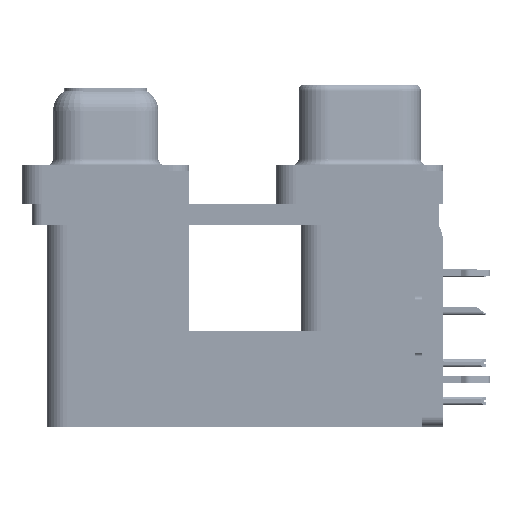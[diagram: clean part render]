
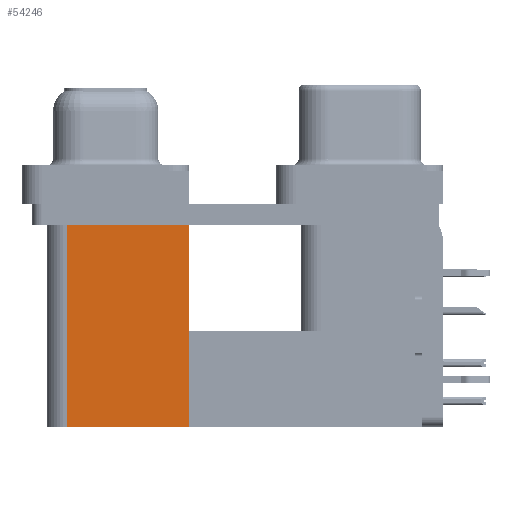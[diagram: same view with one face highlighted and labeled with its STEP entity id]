
A CAD part, left-side view. The second image highlights one B-rep face of the part: STEP entity #54246.
In plain terms, the highlighted planar face has unit normal (-1, 0, 0).
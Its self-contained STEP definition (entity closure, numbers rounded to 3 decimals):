
#5836 = EDGE_CURVE ( 'NONE', #28628, #40779, #12269, .T. ) ;
#7322 = VERTEX_POINT ( 'NONE', #8675 ) ;
#8675 = CARTESIAN_POINT ( 'NONE',  ( 3.7, 21.975, -2.5 ) ) ;
#9451 = CARTESIAN_POINT ( 'NONE',  ( 3.7, 12.775, -19.2 ) ) ;
#10602 = DIRECTION ( 'NONE',  ( 0., 0., 1. ) ) ;
#10950 = DIRECTION ( 'NONE',  ( 0., 1., 0. ) ) ;
#12105 = VECTOR ( 'NONE', #25649, 1000. ) ;
#12132 = PLANE ( 'NONE',  #50577 ) ;
#12269 = LINE ( 'NONE', #42834, #12105 ) ;
#12682 = FACE_OUTER_BOUND ( 'NONE', #15060, .T. ) ;
#15060 = EDGE_LOOP ( 'NONE', ( #32044, #51080, #45745, #30519 ) ) ;
#19413 = LINE ( 'NONE', #32537, #37739 ) ;
#19708 = CARTESIAN_POINT ( 'NONE',  ( 3.7, 12.775, -19.2 ) ) ;
#21911 = CARTESIAN_POINT ( 'NONE',  ( 3.7, 12.775, -2.5 ) ) ;
#23082 = CARTESIAN_POINT ( 'NONE',  ( 3.7, 21.975, -19.2 ) ) ;
#25649 = DIRECTION ( 'NONE',  ( 0., 1., 0. ) ) ;
#28628 = VERTEX_POINT ( 'NONE', #19708 ) ;
#28636 = EDGE_CURVE ( 'NONE', #32108, #7322, #19413, .T. ) ;
#29405 = VECTOR ( 'NONE', #46054, 1000. ) ;
#30519 = ORIENTED_EDGE ( 'NONE', *, *, #41630, .T. ) ;
#32044 = ORIENTED_EDGE ( 'NONE', *, *, #28636, .T. ) ;
#32108 = VERTEX_POINT ( 'NONE', #21911 ) ;
#32537 = CARTESIAN_POINT ( 'NONE',  ( 3.7, 12.775, -2.5 ) ) ;
#33241 = EDGE_CURVE ( 'NONE', #40779, #7322, #37040, .T. ) ;
#37040 = LINE ( 'NONE', #23082, #29405 ) ;
#37739 = VECTOR ( 'NONE', #10950, 1000. ) ;
#40779 = VERTEX_POINT ( 'NONE', #47713 ) ;
#41630 = EDGE_CURVE ( 'NONE', #28628, #32108, #50461, .T. ) ;
#42834 = CARTESIAN_POINT ( 'NONE',  ( 3.7, 12.775, -19.2 ) ) ;
#43524 = DIRECTION ( 'NONE',  ( 0., 0., -1. ) ) ;
#45745 = ORIENTED_EDGE ( 'NONE', *, *, #5836, .F. ) ;
#46054 = DIRECTION ( 'NONE',  ( 0., 0., 1. ) ) ;
#47601 = CARTESIAN_POINT ( 'NONE',  ( 3.7, 12.775, -19.2 ) ) ;
#47713 = CARTESIAN_POINT ( 'NONE',  ( 3.7, 21.975, -19.2 ) ) ;
#48494 = VECTOR ( 'NONE', #10602, 1000. ) ;
#50461 = LINE ( 'NONE', #9451, #48494 ) ;
#50577 = AXIS2_PLACEMENT_3D ( 'NONE', #47601, #52264, #43524 ) ;
#51080 = ORIENTED_EDGE ( 'NONE', *, *, #33241, .F. ) ;
#52264 = DIRECTION ( 'NONE',  ( 1., 0., 0. ) ) ;
#54246 = ADVANCED_FACE ( 'NONE', ( #12682 ), #12132, .F. ) ;
